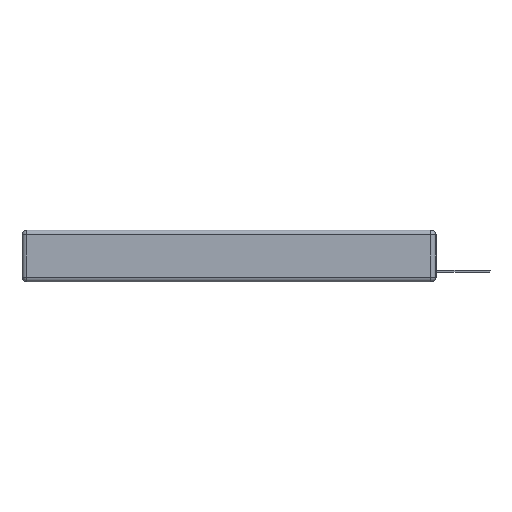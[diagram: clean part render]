
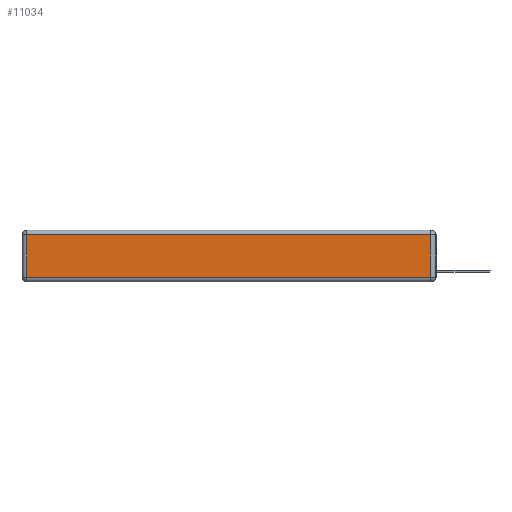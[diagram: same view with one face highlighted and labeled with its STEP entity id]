
A CAD part, left-side view. The second image highlights one B-rep face of the part: STEP entity #11034.
In plain terms, the highlighted planar face has unit normal (-1, 0, 0).
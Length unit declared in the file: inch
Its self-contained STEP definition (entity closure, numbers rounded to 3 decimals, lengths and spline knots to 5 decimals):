
#444 = DIRECTION ( 'NONE',  ( 0., 1., 0. ) ) ;
#548 = EDGE_CURVE ( 'NONE', #10555, #10362, #1543, .T. ) ;
#763 = ORIENTED_EDGE ( 'NONE', *, *, #12030, .T. ) ;
#1036 = CARTESIAN_POINT ( 'NONE',  ( 0., 2.72, -0.343 ) ) ;
#1113 = DIRECTION ( 'NONE',  ( 0., 0., -1. ) ) ;
#1201 = PLANE ( 'NONE',  #5074 ) ;
#1543 = LINE ( 'NONE', #9207, #7405 ) ;
#1622 = EDGE_CURVE ( 'NONE', #10362, #4747, #7792, .T. ) ;
#1669 = EDGE_CURVE ( 'NONE', #6723, #10555, #14404, .T. ) ;
#1938 = EDGE_LOOP ( 'NONE', ( #763, #3814, #6994, #10436 ) ) ;
#1989 = LINE ( 'NONE', #6625, #4394 ) ;
#2300 = CARTESIAN_POINT ( 'NONE',  ( 0., 0., -0.343 ) ) ;
#3333 = DIRECTION ( 'NONE',  ( -1., 0., 0. ) ) ;
#3814 = ORIENTED_EDGE ( 'NONE', *, *, #1669, .T. ) ;
#4345 = CARTESIAN_POINT ( 'NONE',  ( 0., 0.03, -0.343 ) ) ;
#4394 = VECTOR ( 'NONE', #13089, 39.37008 ) ;
#4747 = VERTEX_POINT ( 'NONE', #12222 ) ;
#5074 = AXIS2_PLACEMENT_3D ( 'NONE', #2300, #3333, #9005 ) ;
#5583 = CARTESIAN_POINT ( 'NONE',  ( 0., 0.03, -0.313 ) ) ;
#5817 = CARTESIAN_POINT ( 'NONE',  ( 0., 2.72, -0.03 ) ) ;
#6625 = CARTESIAN_POINT ( 'NONE',  ( 0., 0., -0.313 ) ) ;
#6716 = FACE_OUTER_BOUND ( 'NONE', #1938, .T. ) ;
#6723 = VERTEX_POINT ( 'NONE', #5583 ) ;
#6947 = CARTESIAN_POINT ( 'NONE',  ( 0., 0.03, -0.03 ) ) ;
#6994 = ORIENTED_EDGE ( 'NONE', *, *, #548, .T. ) ;
#7405 = VECTOR ( 'NONE', #444, 39.37008 ) ;
#7792 = LINE ( 'NONE', #1036, #12613 ) ;
#8995 = DIRECTION ( 'NONE',  ( 0., 0., 1. ) ) ;
#9005 = DIRECTION ( 'NONE',  ( 0., 0., 1. ) ) ;
#9207 = CARTESIAN_POINT ( 'NONE',  ( 0., 2.75, -0.03 ) ) ;
#10362 = VERTEX_POINT ( 'NONE', #5817 ) ;
#10436 = ORIENTED_EDGE ( 'NONE', *, *, #1622, .T. ) ;
#10555 = VERTEX_POINT ( 'NONE', #6947 ) ;
#11034 = ADVANCED_FACE ( 'NONE', ( #6716 ), #1201, .T. ) ;
#12030 = EDGE_CURVE ( 'NONE', #4747, #6723, #1989, .T. ) ;
#12222 = CARTESIAN_POINT ( 'NONE',  ( 0., 2.72, -0.313 ) ) ;
#12613 = VECTOR ( 'NONE', #1113, 39.37008 ) ;
#13085 = VECTOR ( 'NONE', #8995, 39.37008 ) ;
#13089 = DIRECTION ( 'NONE',  ( 0., -1., 0. ) ) ;
#14404 = LINE ( 'NONE', #4345, #13085 ) ;
